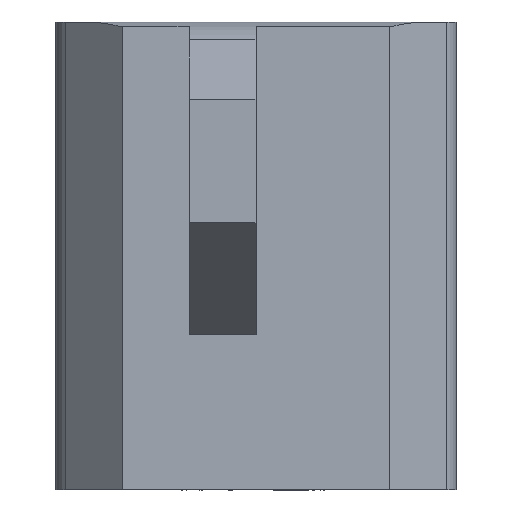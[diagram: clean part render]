
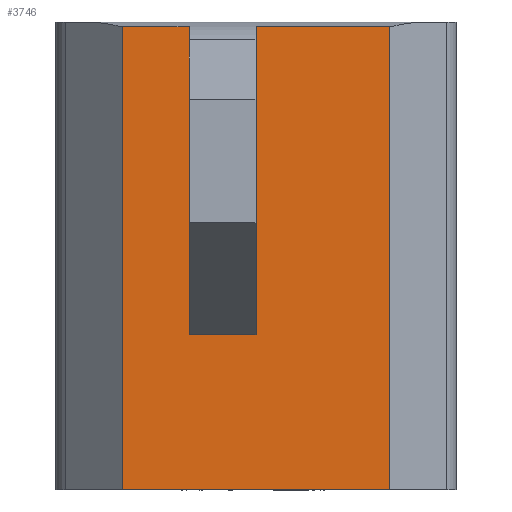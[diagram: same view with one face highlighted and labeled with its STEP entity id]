
A CAD part, front view. The second image highlights one B-rep face of the part: STEP entity #3746.
In plain terms, the highlighted planar face has unit normal (0, -1, 0).
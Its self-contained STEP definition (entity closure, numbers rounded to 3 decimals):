
#202 = LINE ( 'NONE', #4547, #6545 ) ;
#289 = DIRECTION ( 'NONE',  ( 0., 0., -1. ) ) ;
#402 = CARTESIAN_POINT ( 'NONE',  ( 10., -15., 9.634 ) ) ;
#508 = CARTESIAN_POINT ( 'NONE',  ( -10., -15., -15. ) ) ;
#856 = LINE ( 'NONE', #508, #9371 ) ;
#951 = ORIENTED_EDGE ( 'NONE', *, *, #4641, .F. ) ;
#1017 = DIRECTION ( 'NONE',  ( -1., 0., 0. ) ) ;
#1299 = AXIS2_PLACEMENT_3D ( 'NONE', #4383, #5231, #289 ) ;
#1307 = EDGE_LOOP ( 'NONE', ( #7046, #5072, #951, #4424, #8945, #7284, #9832, #8167 ) ) ;
#1514 = CARTESIAN_POINT ( 'NONE',  ( 0., -15., 9.634 ) ) ;
#1633 = LINE ( 'NONE', #3606, #1886 ) ;
#1886 = VECTOR ( 'NONE', #9389, 1000. ) ;
#1939 = VERTEX_POINT ( 'NONE', #6781 ) ;
#1964 = VERTEX_POINT ( 'NONE', #5152 ) ;
#1984 = EDGE_CURVE ( 'NONE', #1964, #3263, #5751, .T. ) ;
#2101 = DIRECTION ( 'NONE',  ( -1., 0., 0. ) ) ;
#2481 = VERTEX_POINT ( 'NONE', #402 ) ;
#3064 = VERTEX_POINT ( 'NONE', #4098 ) ;
#3263 = VERTEX_POINT ( 'NONE', #8583 ) ;
#3606 = CARTESIAN_POINT ( 'NONE',  ( -5., -15., 9.634 ) ) ;
#3746 = ADVANCED_FACE ( 'NONE', ( #7094 ), #9349, .T. ) ;
#3929 = LINE ( 'NONE', #8746, #5894 ) ;
#4098 = CARTESIAN_POINT ( 'NONE',  ( 0., -15., -13.391 ) ) ;
#4383 = CARTESIAN_POINT ( 'NONE',  ( -15., -15., -15. ) ) ;
#4421 = EDGE_CURVE ( 'NONE', #3064, #5050, #5637, .T. ) ;
#4424 = ORIENTED_EDGE ( 'NONE', *, *, #4763, .T. ) ;
#4452 = VECTOR ( 'NONE', #10510, 1000. ) ;
#4547 = CARTESIAN_POINT ( 'NONE',  ( -15., -15., -13.391 ) ) ;
#4641 = EDGE_CURVE ( 'NONE', #8034, #1939, #6824, .T. ) ;
#4763 = EDGE_CURVE ( 'NONE', #8034, #9557, #1633, .T. ) ;
#4920 = EDGE_CURVE ( 'NONE', #9557, #3263, #856, .T. ) ;
#5044 = EDGE_CURVE ( 'NONE', #1964, #2481, #8857, .T. ) ;
#5050 = VERTEX_POINT ( 'NONE', #1514 ) ;
#5072 = ORIENTED_EDGE ( 'NONE', *, *, #9719, .T. ) ;
#5137 = CARTESIAN_POINT ( 'NONE',  ( -10., -15., 9.634 ) ) ;
#5152 = CARTESIAN_POINT ( 'NONE',  ( 10., -15., -25. ) ) ;
#5180 = EDGE_CURVE ( 'NONE', #2481, #5050, #3929, .T. ) ;
#5231 = DIRECTION ( 'NONE',  ( 0., -1., 0. ) ) ;
#5539 = CARTESIAN_POINT ( 'NONE',  ( 0., -15., 9.634 ) ) ;
#5637 = LINE ( 'NONE', #5539, #9760 ) ;
#5751 = LINE ( 'NONE', #7663, #7685 ) ;
#5894 = VECTOR ( 'NONE', #10337, 1000. ) ;
#6327 = DIRECTION ( 'NONE',  ( 0., 0., -1. ) ) ;
#6390 = DIRECTION ( 'NONE',  ( 0., 0., 1. ) ) ;
#6545 = VECTOR ( 'NONE', #2101, 1000. ) ;
#6781 = CARTESIAN_POINT ( 'NONE',  ( -5., -15., -13.391 ) ) ;
#6824 = LINE ( 'NONE', #10669, #8725 ) ;
#7046 = ORIENTED_EDGE ( 'NONE', *, *, #4421, .F. ) ;
#7094 = FACE_OUTER_BOUND ( 'NONE', #1307, .T. ) ;
#7243 = CARTESIAN_POINT ( 'NONE',  ( 10., -15., -15. ) ) ;
#7284 = ORIENTED_EDGE ( 'NONE', *, *, #1984, .F. ) ;
#7663 = CARTESIAN_POINT ( 'NONE',  ( 15., -15., -25. ) ) ;
#7685 = VECTOR ( 'NONE', #1017, 1000. ) ;
#8034 = VERTEX_POINT ( 'NONE', #10496 ) ;
#8167 = ORIENTED_EDGE ( 'NONE', *, *, #5180, .T. ) ;
#8583 = CARTESIAN_POINT ( 'NONE',  ( -10., -15., -25. ) ) ;
#8725 = VECTOR ( 'NONE', #9036, 1000. ) ;
#8746 = CARTESIAN_POINT ( 'NONE',  ( 10., -15., 9.634 ) ) ;
#8857 = LINE ( 'NONE', #7243, #4452 ) ;
#8945 = ORIENTED_EDGE ( 'NONE', *, *, #4920, .T. ) ;
#9036 = DIRECTION ( 'NONE',  ( 0., 0., -1. ) ) ;
#9349 = PLANE ( 'NONE',  #1299 ) ;
#9371 = VECTOR ( 'NONE', #6327, 1000. ) ;
#9389 = DIRECTION ( 'NONE',  ( -1., 0., 0. ) ) ;
#9557 = VERTEX_POINT ( 'NONE', #5137 ) ;
#9719 = EDGE_CURVE ( 'NONE', #3064, #1939, #202, .T. ) ;
#9760 = VECTOR ( 'NONE', #6390, 1000. ) ;
#9832 = ORIENTED_EDGE ( 'NONE', *, *, #5044, .T. ) ;
#10337 = DIRECTION ( 'NONE',  ( -1., 0., 0. ) ) ;
#10496 = CARTESIAN_POINT ( 'NONE',  ( -5., -15., 9.634 ) ) ;
#10510 = DIRECTION ( 'NONE',  ( 0., 0., 1. ) ) ;
#10669 = CARTESIAN_POINT ( 'NONE',  ( -5., -15., -25. ) ) ;
